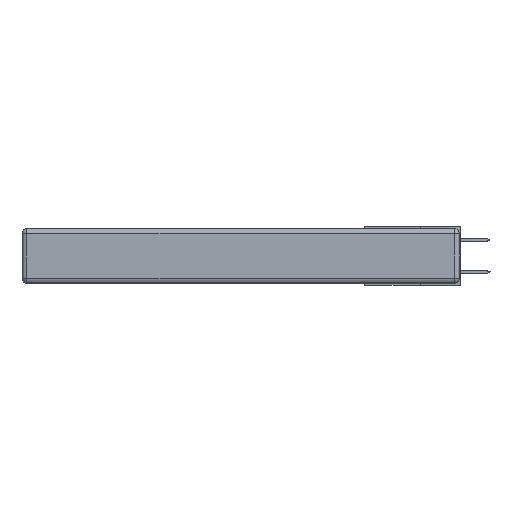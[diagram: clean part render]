
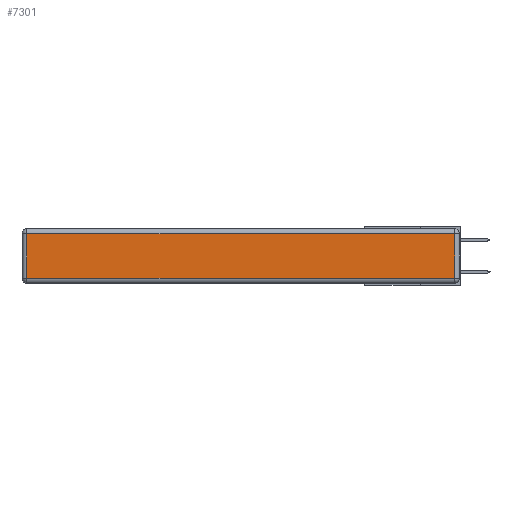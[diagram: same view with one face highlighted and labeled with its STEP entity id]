
A CAD part, left-side view. The second image highlights one B-rep face of the part: STEP entity #7301.
In plain terms, the highlighted planar face has unit normal (-1, 0, 0).
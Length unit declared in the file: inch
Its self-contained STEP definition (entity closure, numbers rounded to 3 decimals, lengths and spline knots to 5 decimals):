
#69 = CARTESIAN_POINT ( 'NONE',  ( 0., 0., -0.313 ) ) ;
#115 = ORIENTED_EDGE ( 'NONE', *, *, #5409, .T. ) ;
#2847 = CARTESIAN_POINT ( 'NONE',  ( 0., 0.03, -0.03 ) ) ;
#3772 = DIRECTION ( 'NONE',  ( 0., 1., 0. ) ) ;
#4398 = LINE ( 'NONE', #69, #11083 ) ;
#4513 = VECTOR ( 'NONE', #12603, 39.37008 ) ;
#4870 = CARTESIAN_POINT ( 'NONE',  ( 0., 2.72, -0.313 ) ) ;
#5118 = VECTOR ( 'NONE', #7258, 39.37008 ) ;
#5287 = CARTESIAN_POINT ( 'NONE',  ( 0., 0.03, -0.343 ) ) ;
#5409 = EDGE_CURVE ( 'NONE', #10472, #11058, #11474, .T. ) ;
#7147 = EDGE_CURVE ( 'NONE', #12996, #12582, #4398, .T. ) ;
#7177 = AXIS2_PLACEMENT_3D ( 'NONE', #8155, #9298, #7240 ) ;
#7240 = DIRECTION ( 'NONE',  ( 0., 0., 1. ) ) ;
#7258 = DIRECTION ( 'NONE',  ( 0., 0., 1. ) ) ;
#7301 = ADVANCED_FACE ( 'NONE', ( #10742 ), #13673, .T. ) ;
#7548 = CARTESIAN_POINT ( 'NONE',  ( 0., 0.03, -0.313 ) ) ;
#7761 = DIRECTION ( 'NONE',  ( 0., -1., 0. ) ) ;
#8155 = CARTESIAN_POINT ( 'NONE',  ( 0., 0., -0.343 ) ) ;
#8537 = VECTOR ( 'NONE', #3772, 39.37008 ) ;
#8814 = EDGE_CURVE ( 'NONE', #12582, #10472, #10944, .T. ) ;
#8873 = EDGE_LOOP ( 'NONE', ( #9399, #11949, #115, #9038 ) ) ;
#9038 = ORIENTED_EDGE ( 'NONE', *, *, #12210, .T. ) ;
#9298 = DIRECTION ( 'NONE',  ( -1., 0., 0. ) ) ;
#9312 = LINE ( 'NONE', #10152, #4513 ) ;
#9399 = ORIENTED_EDGE ( 'NONE', *, *, #7147, .T. ) ;
#10152 = CARTESIAN_POINT ( 'NONE',  ( 0., 2.72, -0.343 ) ) ;
#10472 = VERTEX_POINT ( 'NONE', #2847 ) ;
#10742 = FACE_OUTER_BOUND ( 'NONE', #8873, .T. ) ;
#10944 = LINE ( 'NONE', #5287, #5118 ) ;
#11058 = VERTEX_POINT ( 'NONE', #11679 ) ;
#11083 = VECTOR ( 'NONE', #7761, 39.37008 ) ;
#11474 = LINE ( 'NONE', #11520, #8537 ) ;
#11520 = CARTESIAN_POINT ( 'NONE',  ( 0., 2.75, -0.03 ) ) ;
#11679 = CARTESIAN_POINT ( 'NONE',  ( 0., 2.72, -0.03 ) ) ;
#11949 = ORIENTED_EDGE ( 'NONE', *, *, #8814, .T. ) ;
#12210 = EDGE_CURVE ( 'NONE', #11058, #12996, #9312, .T. ) ;
#12582 = VERTEX_POINT ( 'NONE', #7548 ) ;
#12603 = DIRECTION ( 'NONE',  ( 0., 0., -1. ) ) ;
#12996 = VERTEX_POINT ( 'NONE', #4870 ) ;
#13673 = PLANE ( 'NONE',  #7177 ) ;
